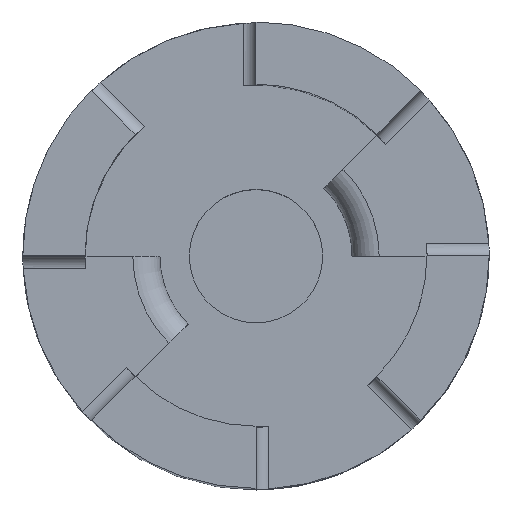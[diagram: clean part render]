
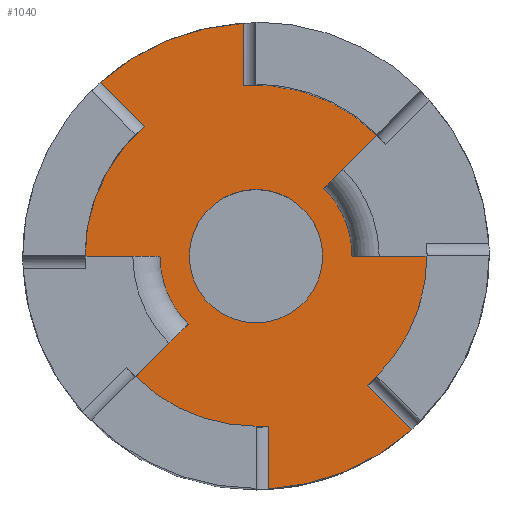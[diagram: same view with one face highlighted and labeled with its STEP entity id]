
A CAD part, top view. The second image highlights one B-rep face of the part: STEP entity #1040.
In plain terms, the highlighted planar face has unit normal (0, 0, 1).
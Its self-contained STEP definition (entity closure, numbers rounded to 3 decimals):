
#29=FACE_BOUND('',#172,.T.);
#65=PLANE('',#1160);
#114=FACE_OUTER_BOUND('',#171,.T.);
#171=EDGE_LOOP('',(#872,#873,#874,#875,#876,#877,#878,#879,#880,#881,#882,
#883,#884,#885,#886,#887));
#172=EDGE_LOOP('',(#888));
#195=LINE('',#1518,#279);
#202=LINE('',#1547,#286);
#251=LINE('',#1851,#335);
#254=LINE('',#1869,#338);
#256=LINE('',#1875,#340);
#257=LINE('',#1879,#341);
#258=LINE('',#1881,#342);
#259=LINE('',#1885,#343);
#279=VECTOR('',#1213,10.);
#286=VECTOR('',#1240,10.);
#335=VECTOR('',#1407,10.);
#338=VECTOR('',#1414,10.);
#340=VECTOR('',#1420,10.);
#341=VECTOR('',#1425,10.);
#342=VECTOR('',#1426,10.);
#343=VECTOR('',#1429,10.);
#360=CIRCLE('',#1081,3.125);
#377=CIRCLE('',#1111,10.922);
#385=CIRCLE('',#1119,10.922);
#405=CIRCLE('',#1161,8.01);
#406=CIRCLE('',#1162,4.5);
#407=CIRCLE('',#1163,8.01);
#408=CIRCLE('',#1164,8.01);
#409=CIRCLE('',#1165,4.5);
#410=CIRCLE('',#1166,8.01);
#415=VERTEX_POINT('',#1498);
#422=VERTEX_POINT('',#1515);
#423=VERTEX_POINT('',#1517);
#434=VERTEX_POINT('',#1544);
#435=VERTEX_POINT('',#1546);
#455=VERTEX_POINT('',#1674);
#456=VERTEX_POINT('',#1685);
#471=VERTEX_POINT('',#1726);
#472=VERTEX_POINT('',#1737);
#500=VERTEX_POINT('',#1838);
#504=VERTEX_POINT('',#1858);
#505=VERTEX_POINT('',#1872);
#506=VERTEX_POINT('',#1874);
#507=VERTEX_POINT('',#1877);
#508=VERTEX_POINT('',#1880);
#509=VERTEX_POINT('',#1882);
#510=VERTEX_POINT('',#1884);
#518=EDGE_CURVE('',#415,#415,#360,.T.);
#527=EDGE_CURVE('',#423,#422,#195,.T.);
#541=EDGE_CURVE('',#435,#434,#202,.T.);
#570=EDGE_CURVE('',#456,#455,#377,.F.);
#588=EDGE_CURVE('',#472,#471,#385,.F.);
#635=EDGE_CURVE('',#472,#500,#251,.T.);
#639=EDGE_CURVE('',#504,#471,#254,.T.);
#641=EDGE_CURVE('',#504,#505,#405,.T.);
#642=EDGE_CURVE('',#505,#506,#256,.T.);
#643=EDGE_CURVE('',#435,#506,#406,.T.);
#644=EDGE_CURVE('',#434,#507,#407,.T.);
#645=EDGE_CURVE('',#456,#507,#257,.T.);
#646=EDGE_CURVE('',#508,#455,#258,.T.);
#647=EDGE_CURVE('',#508,#509,#408,.T.);
#648=EDGE_CURVE('',#509,#510,#259,.T.);
#649=EDGE_CURVE('',#423,#510,#409,.T.);
#650=EDGE_CURVE('',#422,#500,#410,.T.);
#872=ORIENTED_EDGE('',*,*,#635,.F.);
#873=ORIENTED_EDGE('',*,*,#588,.T.);
#874=ORIENTED_EDGE('',*,*,#639,.F.);
#875=ORIENTED_EDGE('',*,*,#641,.T.);
#876=ORIENTED_EDGE('',*,*,#642,.T.);
#877=ORIENTED_EDGE('',*,*,#643,.F.);
#878=ORIENTED_EDGE('',*,*,#541,.T.);
#879=ORIENTED_EDGE('',*,*,#644,.T.);
#880=ORIENTED_EDGE('',*,*,#645,.F.);
#881=ORIENTED_EDGE('',*,*,#570,.T.);
#882=ORIENTED_EDGE('',*,*,#646,.F.);
#883=ORIENTED_EDGE('',*,*,#647,.T.);
#884=ORIENTED_EDGE('',*,*,#648,.T.);
#885=ORIENTED_EDGE('',*,*,#649,.F.);
#886=ORIENTED_EDGE('',*,*,#527,.T.);
#887=ORIENTED_EDGE('',*,*,#650,.T.);
#888=ORIENTED_EDGE('',*,*,#518,.T.);
#1040=ADVANCED_FACE('',(#114,#29),#65,.T.);
#1081=AXIS2_PLACEMENT_3D('',#1499,#1194,#1195);
#1111=AXIS2_PLACEMENT_3D('',#1686,#1280,#1281);
#1119=AXIS2_PLACEMENT_3D('',#1738,#1304,#1305);
#1160=AXIS2_PLACEMENT_3D('',#1871,#1416,#1417);
#1161=AXIS2_PLACEMENT_3D('',#1873,#1418,#1419);
#1162=AXIS2_PLACEMENT_3D('',#1876,#1421,#1422);
#1163=AXIS2_PLACEMENT_3D('',#1878,#1423,#1424);
#1164=AXIS2_PLACEMENT_3D('',#1883,#1427,#1428);
#1165=AXIS2_PLACEMENT_3D('',#1886,#1430,#1431);
#1166=AXIS2_PLACEMENT_3D('',#1887,#1432,#1433);
#1194=DIRECTION('center_axis',(0.,0.,-1.));
#1195=DIRECTION('ref_axis',(1.,0.,0.));
#1213=DIRECTION('',(0.707,0.707,0.));
#1240=DIRECTION('',(-0.707,-0.707,0.));
#1280=DIRECTION('center_axis',(0.,0.,-1.));
#1281=DIRECTION('ref_axis',(1.,0.,0.));
#1304=DIRECTION('center_axis',(0.,0.,-1.));
#1305=DIRECTION('ref_axis',(1.,0.,0.));
#1407=DIRECTION('',(0.,-1.,0.));
#1414=DIRECTION('',(-0.707,0.707,0.));
#1416=DIRECTION('center_axis',(0.,0.,1.));
#1417=DIRECTION('ref_axis',(1.,0.,0.));
#1418=DIRECTION('center_axis',(0.,0.,1.));
#1419=DIRECTION('ref_axis',(0.707,-0.707,0.));
#1420=DIRECTION('',(1.,0.,0.));
#1421=DIRECTION('center_axis',(0.,0.,-1.));
#1422=DIRECTION('ref_axis',(1.,0.,0.));
#1423=DIRECTION('center_axis',(0.,0.,1.));
#1424=DIRECTION('ref_axis',(0.707,-0.707,0.));
#1425=DIRECTION('',(0.,1.,0.));
#1426=DIRECTION('',(0.707,-0.707,0.));
#1427=DIRECTION('center_axis',(0.,0.,1.));
#1428=DIRECTION('ref_axis',(-0.707,0.707,0.));
#1429=DIRECTION('',(-1.,0.,0.));
#1430=DIRECTION('center_axis',(0.,0.,-1.));
#1431=DIRECTION('ref_axis',(1.,0.,0.));
#1432=DIRECTION('center_axis',(0.,0.,1.));
#1433=DIRECTION('ref_axis',(-0.707,0.707,0.));
#1498=CARTESIAN_POINT('',(-3.125,0.,2.54));
#1499=CARTESIAN_POINT('Origin',(0.,0.,2.54));
#1515=CARTESIAN_POINT('',(5.664,5.664,2.54));
#1517=CARTESIAN_POINT('',(3.182,3.182,2.54));
#1518=CARTESIAN_POINT('',(2.832,2.832,2.54));
#1544=CARTESIAN_POINT('',(-5.664,-5.664,2.54));
#1546=CARTESIAN_POINT('',(-3.182,-3.182,2.54));
#1547=CARTESIAN_POINT('',(-2.832,-2.832,2.54));
#1674=CARTESIAN_POINT('',(7.287,-8.136,2.54));
#1685=CARTESIAN_POINT('',(0.6,-10.906,2.54));
#1686=CARTESIAN_POINT('Origin',(0.,0.,2.54));
#1726=CARTESIAN_POINT('',(-7.287,8.136,2.54));
#1737=CARTESIAN_POINT('',(-0.6,10.906,2.54));
#1738=CARTESIAN_POINT('Origin',(0.,0.,2.54));
#1838=CARTESIAN_POINT('',(-0.6,7.987,2.54));
#1851=CARTESIAN_POINT('',(-0.6,5.08,2.54));
#1858=CARTESIAN_POINT('',(-5.224,6.072,2.54));
#1869=CARTESIAN_POINT('',(-2.408,3.256,2.54));
#1871=CARTESIAN_POINT('Origin',(0.,0.,
2.54));
#1872=CARTESIAN_POINT('',(-8.01,0.,2.54));
#1873=CARTESIAN_POINT('Origin',(0.,0.,
2.54));
#1874=CARTESIAN_POINT('',(-4.5,0.,2.54));
#1875=CARTESIAN_POINT('',(-1.594,0.,2.54));
#1876=CARTESIAN_POINT('Origin',(0.,0.,2.54));
#1877=CARTESIAN_POINT('',(0.6,-7.987,2.54));
#1878=CARTESIAN_POINT('Origin',(0.,0.,
2.54));
#1879=CARTESIAN_POINT('',(0.6,-5.08,2.54));
#1880=CARTESIAN_POINT('',(5.224,-6.072,2.54));
#1881=CARTESIAN_POINT('',(2.408,-3.256,2.54));
#1882=CARTESIAN_POINT('',(8.01,0.,2.54));
#1883=CARTESIAN_POINT('Origin',(0.,0.,
2.54));
#1884=CARTESIAN_POINT('',(4.5,0.,2.54));
#1885=CARTESIAN_POINT('',(1.594,0.,2.54));
#1886=CARTESIAN_POINT('Origin',(0.,0.,2.54));
#1887=CARTESIAN_POINT('Origin',(0.,0.,
2.54));
